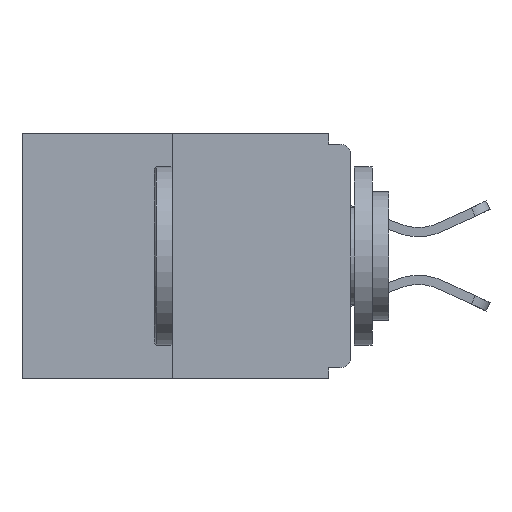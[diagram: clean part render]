
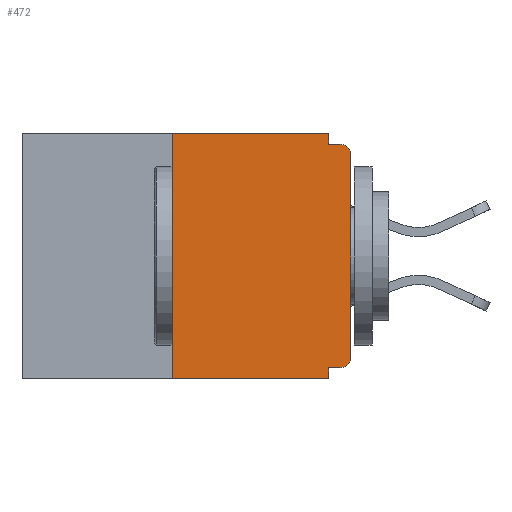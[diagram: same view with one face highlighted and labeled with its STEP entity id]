
A CAD part, left-side view. The second image highlights one B-rep face of the part: STEP entity #472.
In plain terms, the highlighted planar face has unit normal (-1, 0, 0).
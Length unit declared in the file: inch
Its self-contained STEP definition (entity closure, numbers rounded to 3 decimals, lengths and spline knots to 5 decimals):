
#103 = DIRECTION ( 'NONE',  ( 1., 0., 0. ) ) ;
#160 = LINE ( 'NONE', #9569, #19047 ) ;
#472 = ADVANCED_FACE ( 'NONE', ( #6442 ), #9293, .F. ) ;
#951 = CARTESIAN_POINT ( 'NONE',  ( 0., 0., -0.313 ) ) ;
#1274 = CARTESIAN_POINT ( 'NONE',  ( 0., 0.015, -0.015 ) ) ;
#1455 = ORIENTED_EDGE ( 'NONE', *, *, #7110, .F. ) ;
#2709 = VECTOR ( 'NONE', #4392, 39.37008 ) ;
#2723 = ORIENTED_EDGE ( 'NONE', *, *, #16716, .F. ) ;
#2942 = CARTESIAN_POINT ( 'NONE',  ( 0., 0.015, -0.313 ) ) ;
#3045 = DIRECTION ( 'NONE',  ( 0., -1., 0. ) ) ;
#3138 = EDGE_CURVE ( 'NONE', #23481, #9169, #14019, .T. ) ;
#3735 = CARTESIAN_POINT ( 'NONE',  ( 0., 0.031, -0.328 ) ) ;
#4176 = ORIENTED_EDGE ( 'NONE', *, *, #6633, .F. ) ;
#4239 = VERTEX_POINT ( 'NONE', #22286 ) ;
#4392 = DIRECTION ( 'NONE',  ( 0., 0., -1. ) ) ;
#4520 = VECTOR ( 'NONE', #20660, 39.37008 ) ;
#4722 = VERTEX_POINT ( 'NONE', #951 ) ;
#4781 = DIRECTION ( 'NONE',  ( -1., 0., 0. ) ) ;
#5238 = VERTEX_POINT ( 'NONE', #8676 ) ;
#5758 = LINE ( 'NONE', #10667, #20046 ) ;
#6159 = CARTESIAN_POINT ( 'NONE',  ( 0., 0.25, 0. ) ) ;
#6269 = EDGE_CURVE ( 'NONE', #5238, #13434, #160, .T. ) ;
#6442 = FACE_OUTER_BOUND ( 'NONE', #12071, .T. ) ;
#6493 = CARTESIAN_POINT ( 'NONE',  ( 0., 0.031, -0.343 ) ) ;
#6633 = EDGE_CURVE ( 'NONE', #20865, #13796, #12749, .T. ) ;
#7110 = EDGE_CURVE ( 'NONE', #4239, #7933, #7609, .T. ) ;
#7376 = DIRECTION ( 'NONE',  ( 0., 0., -1. ) ) ;
#7609 = LINE ( 'NONE', #7788, #2709 ) ;
#7788 = CARTESIAN_POINT ( 'NONE',  ( 0., 0.031, 0. ) ) ;
#7791 = CARTESIAN_POINT ( 'NONE',  ( 0., 0., 0. ) ) ;
#7840 = CIRCLE ( 'NONE', #17739, 0.015 ) ;
#7912 = CARTESIAN_POINT ( 'NONE',  ( 0., 0., -0.328 ) ) ;
#7933 = VERTEX_POINT ( 'NONE', #18307 ) ;
#8646 = ORIENTED_EDGE ( 'NONE', *, *, #21489, .T. ) ;
#8676 = CARTESIAN_POINT ( 'NONE',  ( 0., 0.25, -0.343 ) ) ;
#8900 = ORIENTED_EDGE ( 'NONE', *, *, #17106, .F. ) ;
#9169 = VERTEX_POINT ( 'NONE', #1274 ) ;
#9293 = PLANE ( 'NONE',  #12124 ) ;
#9350 = CARTESIAN_POINT ( 'NONE',  ( 0., 0.46, 0. ) ) ;
#9376 = ORIENTED_EDGE ( 'NONE', *, *, #17513, .F. ) ;
#9569 = CARTESIAN_POINT ( 'NONE',  ( 0., 0.46, -0.343 ) ) ;
#9827 = CARTESIAN_POINT ( 'NONE',  ( 0., 0.031, -0.343 ) ) ;
#10172 = CARTESIAN_POINT ( 'NONE',  ( 0., 0.015, -0.03 ) ) ;
#10183 = LINE ( 'NONE', #7791, #4520 ) ;
#10667 = CARTESIAN_POINT ( 'NONE',  ( 0., 0., -0.015 ) ) ;
#11117 = LINE ( 'NONE', #6493, #12252 ) ;
#11303 = VERTEX_POINT ( 'NONE', #6159 ) ;
#11964 = DIRECTION ( 'NONE',  ( 0., 0., -1. ) ) ;
#12034 = EDGE_CURVE ( 'NONE', #4722, #23481, #10183, .T. ) ;
#12071 = EDGE_LOOP ( 'NONE', ( #18762, #8900, #21925, #9376, #4176, #8646, #21149, #19657, #2723, #1455 ) ) ;
#12124 = AXIS2_PLACEMENT_3D ( 'NONE', #18345, #103, #7376 ) ;
#12252 = VECTOR ( 'NONE', #18371, 39.37008 ) ;
#12749 = LINE ( 'NONE', #7912, #14753 ) ;
#13434 = VERTEX_POINT ( 'NONE', #9827 ) ;
#13796 = VERTEX_POINT ( 'NONE', #3735 ) ;
#13922 = DIRECTION ( 'NONE',  ( -1., 0., 0. ) ) ;
#14019 = CIRCLE ( 'NONE', #14099, 0.015 ) ;
#14099 = AXIS2_PLACEMENT_3D ( 'NONE', #10172, #4781, #11964 ) ;
#14382 = LINE ( 'NONE', #9350, #18703 ) ;
#14753 = VECTOR ( 'NONE', #20620, 39.37008 ) ;
#15608 = EDGE_CURVE ( 'NONE', #11303, #4239, #14382, .T. ) ;
#16602 = VECTOR ( 'NONE', #19788, 39.37008 ) ;
#16716 = EDGE_CURVE ( 'NONE', #7933, #9169, #5758, .T. ) ;
#17106 = EDGE_CURVE ( 'NONE', #5238, #11303, #21457, .T. ) ;
#17513 = EDGE_CURVE ( 'NONE', #13796, #13434, #11117, .T. ) ;
#17739 = AXIS2_PLACEMENT_3D ( 'NONE', #2942, #13922, #21361 ) ;
#18307 = CARTESIAN_POINT ( 'NONE',  ( 0., 0.031, -0.015 ) ) ;
#18345 = CARTESIAN_POINT ( 'NONE',  ( 0., 0.46, 0. ) ) ;
#18371 = DIRECTION ( 'NONE',  ( 0., 0., -1. ) ) ;
#18590 = CARTESIAN_POINT ( 'NONE',  ( 0., 0.015, -0.328 ) ) ;
#18703 = VECTOR ( 'NONE', #22724, 39.37008 ) ;
#18762 = ORIENTED_EDGE ( 'NONE', *, *, #15608, .F. ) ;
#19047 = VECTOR ( 'NONE', #21390, 39.37008 ) ;
#19538 = CARTESIAN_POINT ( 'NONE',  ( 0., 0.25, 0. ) ) ;
#19657 = ORIENTED_EDGE ( 'NONE', *, *, #3138, .T. ) ;
#19788 = DIRECTION ( 'NONE',  ( 0., 0., 1. ) ) ;
#20046 = VECTOR ( 'NONE', #3045, 39.37008 ) ;
#20620 = DIRECTION ( 'NONE',  ( 0., 1., 0. ) ) ;
#20660 = DIRECTION ( 'NONE',  ( 0., 0., 1. ) ) ;
#20865 = VERTEX_POINT ( 'NONE', #18590 ) ;
#21149 = ORIENTED_EDGE ( 'NONE', *, *, #12034, .T. ) ;
#21361 = DIRECTION ( 'NONE',  ( 0., 0., -1. ) ) ;
#21390 = DIRECTION ( 'NONE',  ( 0., -1., 0. ) ) ;
#21457 = LINE ( 'NONE', #19538, #16602 ) ;
#21489 = EDGE_CURVE ( 'NONE', #20865, #4722, #7840, .T. ) ;
#21579 = CARTESIAN_POINT ( 'NONE',  ( 0., 0., -0.03 ) ) ;
#21925 = ORIENTED_EDGE ( 'NONE', *, *, #6269, .T. ) ;
#22286 = CARTESIAN_POINT ( 'NONE',  ( 0., 0.031, 0. ) ) ;
#22724 = DIRECTION ( 'NONE',  ( 0., -1., 0. ) ) ;
#23481 = VERTEX_POINT ( 'NONE', #21579 ) ;
